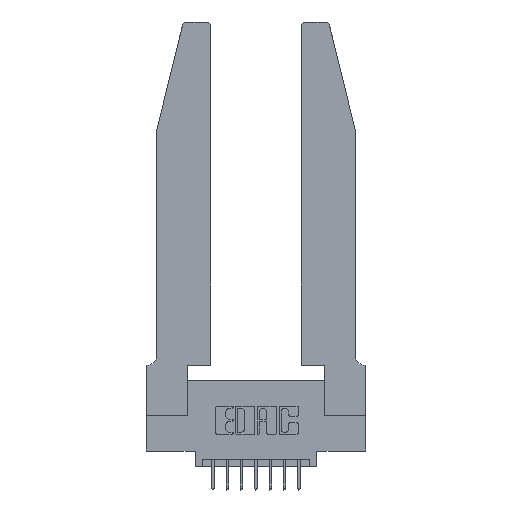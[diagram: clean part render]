
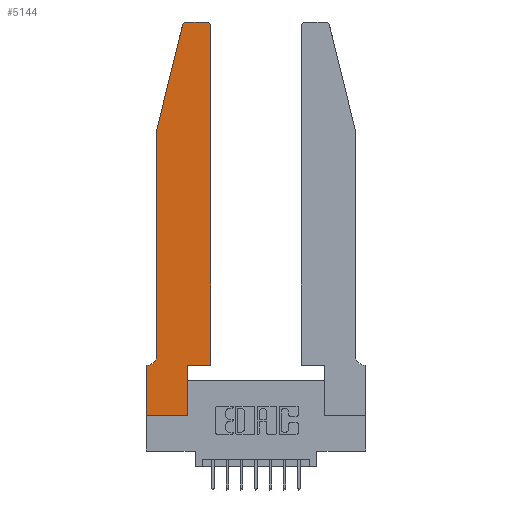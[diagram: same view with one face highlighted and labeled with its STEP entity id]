
A CAD part, top view. The second image highlights one B-rep face of the part: STEP entity #5144.
In plain terms, the highlighted planar face has unit normal (0, 0, 1).
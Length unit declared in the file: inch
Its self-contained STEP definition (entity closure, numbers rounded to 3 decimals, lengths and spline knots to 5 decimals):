
#22 = CIRCLE ( 'NONE', #120, 0.03 ) ;
#120 = AXIS2_PLACEMENT_3D ( 'NONE', #4588, #12678, #5782 ) ;
#139 = ORIENTED_EDGE ( 'NONE', *, *, #5572, .T. ) ;
#431 = CARTESIAN_POINT ( 'NONE',  ( 0.0755, 2., 0.37 ) ) ;
#478 = ORIENTED_EDGE ( 'NONE', *, *, #3799, .T. ) ;
#675 = CARTESIAN_POINT ( 'NONE',  ( 0.2605, 2.75, 0.37 ) ) ;
#695 = DIRECTION ( 'NONE',  ( 1., 0., 0. ) ) ;
#829 = CARTESIAN_POINT ( 'NONE',  ( 0.0055, 0.35, 0.37 ) ) ;
#919 = VERTEX_POINT ( 'NONE', #6341 ) ;
#1049 = LINE ( 'NONE', #13442, #7341 ) ;
#1367 = VECTOR ( 'NONE', #1520, 39.37008 ) ;
#1450 = VECTOR ( 'NONE', #6138, 39.37008 ) ;
#1461 = EDGE_CURVE ( 'NONE', #6743, #2967, #4701, .T. ) ;
#1520 = DIRECTION ( 'NONE',  ( 1., 0., 0. ) ) ;
#1658 = VECTOR ( 'NONE', #6116, 39.37008 ) ;
#1708 = ORIENTED_EDGE ( 'NONE', *, *, #1461, .T. ) ;
#1883 = DIRECTION ( 'NONE',  ( -1., 0., 0. ) ) ;
#2003 = PLANE ( 'NONE',  #6928 ) ;
#2149 = CARTESIAN_POINT ( 'NONE',  ( 0.0055, 0.42, 0.37 ) ) ;
#2235 = VERTEX_POINT ( 'NONE', #829 ) ;
#2285 = CARTESIAN_POINT ( 'NONE',  ( 0.0755, 0.35, 0.37 ) ) ;
#2357 = ORIENTED_EDGE ( 'NONE', *, *, #6143, .T. ) ;
#2608 = LINE ( 'NONE', #5036, #5454 ) ;
#2627 = VERTEX_POINT ( 'NONE', #14366 ) ;
#2683 = VERTEX_POINT ( 'NONE', #5269 ) ;
#2861 = DIRECTION ( 'NONE',  ( 0., -1., 0. ) ) ;
#2967 = VERTEX_POINT ( 'NONE', #8318 ) ;
#3020 = LINE ( 'NONE', #9087, #11970 ) ;
#3148 = VERTEX_POINT ( 'NONE', #5202 ) ;
#3242 = DIRECTION ( 'NONE',  ( 1., 0., 0. ) ) ;
#3246 = EDGE_CURVE ( 'NONE', #3148, #8738, #5780, .T. ) ;
#3302 = CARTESIAN_POINT ( 'NONE',  ( 0.4205, 2.75, 0.37 ) ) ;
#3381 = DIRECTION ( 'NONE',  ( -1., 0., 0. ) ) ;
#3758 = CARTESIAN_POINT ( 'NONE',  ( 0., 0., 0.37 ) ) ;
#3799 = EDGE_CURVE ( 'NONE', #4580, #2683, #1049, .T. ) ;
#4416 = CARTESIAN_POINT ( 'NONE',  ( 0.25487, 2.72718, 0.37 ) ) ;
#4417 = FACE_OUTER_BOUND ( 'NONE', #4481, .T. ) ;
#4481 = EDGE_LOOP ( 'NONE', ( #11755, #11967, #5106, #11023, #139, #14168, #1708, #14652, #2357, #11649, #478, #7758 ) ) ;
#4580 = VERTEX_POINT ( 'NONE', #11398 ) ;
#4588 = CARTESIAN_POINT ( 'NONE',  ( 0.4205, 2.72, 0.37 ) ) ;
#4603 = LINE ( 'NONE', #6350, #1367 ) ;
#4609 = VERTEX_POINT ( 'NONE', #3302 ) ;
#4701 = LINE ( 'NONE', #3758, #1450 ) ;
#4926 = LINE ( 'NONE', #431, #11407 ) ;
#5036 = CARTESIAN_POINT ( 'NONE',  ( 0., 0., 0.37 ) ) ;
#5106 = ORIENTED_EDGE ( 'NONE', *, *, #7364, .T. ) ;
#5144 = ADVANCED_FACE ( 'NONE', ( #4417 ), #2003, .T. ) ;
#5146 = VECTOR ( 'NONE', #1883, 39.37008 ) ;
#5202 = CARTESIAN_POINT ( 'NONE',  ( 0.284, 2.75, 0.37 ) ) ;
#5269 = CARTESIAN_POINT ( 'NONE',  ( 0.4505, 2.72, 0.37 ) ) ;
#5372 = EDGE_CURVE ( 'NONE', #9985, #4580, #4603, .T. ) ;
#5454 = VECTOR ( 'NONE', #13157, 39.37008 ) ;
#5572 = EDGE_CURVE ( 'NONE', #10109, #2235, #8562, .T. ) ;
#5780 = CIRCLE ( 'NONE', #8612, 0.03 ) ;
#5782 = DIRECTION ( 'NONE',  ( 1., 0., 0. ) ) ;
#5936 = CARTESIAN_POINT ( 'NONE',  ( 0.0755, 0.42, 0.37 ) ) ;
#6095 = EDGE_CURVE ( 'NONE', #4609, #3148, #6230, .T. ) ;
#6116 = DIRECTION ( 'NONE',  ( -1., 0., 0. ) ) ;
#6138 = DIRECTION ( 'NONE',  ( 0., -1., 0. ) ) ;
#6143 = EDGE_CURVE ( 'NONE', #919, #9985, #10533, .T. ) ;
#6230 = LINE ( 'NONE', #675, #5146 ) ;
#6243 = EDGE_CURVE ( 'NONE', #2683, #4609, #22, .T. ) ;
#6341 = CARTESIAN_POINT ( 'NONE',  ( 0.2865, 0., 0.37 ) ) ;
#6350 = CARTESIAN_POINT ( 'NONE',  ( 0.4505, 0.35, 0.37 ) ) ;
#6551 = DIRECTION ( 'NONE',  ( 0., 1., 0. ) ) ;
#6733 = DIRECTION ( 'NONE',  ( 0., 1., 0. ) ) ;
#6743 = VERTEX_POINT ( 'NONE', #10212 ) ;
#6800 = DIRECTION ( 'NONE',  ( -0.239, -0.971, 0. ) ) ;
#6928 = AXIS2_PLACEMENT_3D ( 'NONE', #11331, #10206, #3242 ) ;
#7223 = EDGE_CURVE ( 'NONE', #2627, #10109, #4926, .T. ) ;
#7341 = VECTOR ( 'NONE', #6551, 39.37008 ) ;
#7364 = EDGE_CURVE ( 'NONE', #8738, #2627, #3020, .T. ) ;
#7470 = VECTOR ( 'NONE', #6733, 39.37008 ) ;
#7758 = ORIENTED_EDGE ( 'NONE', *, *, #6243, .T. ) ;
#7791 = DIRECTION ( 'NONE',  ( 0., 0., 1. ) ) ;
#7877 = CARTESIAN_POINT ( 'NONE',  ( 0.2865, 0.35, 0.37 ) ) ;
#8318 = CARTESIAN_POINT ( 'NONE',  ( 0., 0., 0.37 ) ) ;
#8562 = CIRCLE ( 'NONE', #15124, 0.07 ) ;
#8612 = AXIS2_PLACEMENT_3D ( 'NONE', #14697, #7791, #695 ) ;
#8738 = VERTEX_POINT ( 'NONE', #4416 ) ;
#9087 = CARTESIAN_POINT ( 'NONE',  ( 0.0755, 2., 0.37 ) ) ;
#9570 = LINE ( 'NONE', #2285, #1658 ) ;
#9985 = VERTEX_POINT ( 'NONE', #7877 ) ;
#10079 = CARTESIAN_POINT ( 'NONE',  ( 0.2865, 0.35, 0.37 ) ) ;
#10109 = VERTEX_POINT ( 'NONE', #5936 ) ;
#10206 = DIRECTION ( 'NONE',  ( 0., 0., 1. ) ) ;
#10212 = CARTESIAN_POINT ( 'NONE',  ( 0., 0.35, 0.37 ) ) ;
#10349 = DIRECTION ( 'NONE',  ( 0., 0., -1. ) ) ;
#10533 = LINE ( 'NONE', #10079, #7470 ) ;
#10881 = EDGE_CURVE ( 'NONE', #2235, #6743, #9570, .T. ) ;
#10948 = EDGE_CURVE ( 'NONE', #2967, #919, #2608, .T. ) ;
#11023 = ORIENTED_EDGE ( 'NONE', *, *, #7223, .T. ) ;
#11331 = CARTESIAN_POINT ( 'NONE',  ( 0., 0.35, 0.37 ) ) ;
#11398 = CARTESIAN_POINT ( 'NONE',  ( 0.4505, 0.35, 0.37 ) ) ;
#11407 = VECTOR ( 'NONE', #2861, 39.37008 ) ;
#11649 = ORIENTED_EDGE ( 'NONE', *, *, #5372, .T. ) ;
#11755 = ORIENTED_EDGE ( 'NONE', *, *, #6095, .T. ) ;
#11967 = ORIENTED_EDGE ( 'NONE', *, *, #3246, .T. ) ;
#11970 = VECTOR ( 'NONE', #6800, 39.37008 ) ;
#12678 = DIRECTION ( 'NONE',  ( 0., 0., 1. ) ) ;
#13157 = DIRECTION ( 'NONE',  ( 1., 0., 0. ) ) ;
#13442 = CARTESIAN_POINT ( 'NONE',  ( 0.4505, 0.35, 0.37 ) ) ;
#14168 = ORIENTED_EDGE ( 'NONE', *, *, #10881, .T. ) ;
#14366 = CARTESIAN_POINT ( 'NONE',  ( 0.0755, 2., 0.37 ) ) ;
#14652 = ORIENTED_EDGE ( 'NONE', *, *, #10948, .T. ) ;
#14697 = CARTESIAN_POINT ( 'NONE',  ( 0.284, 2.72, 0.37 ) ) ;
#15124 = AXIS2_PLACEMENT_3D ( 'NONE', #2149, #10349, #3381 ) ;
